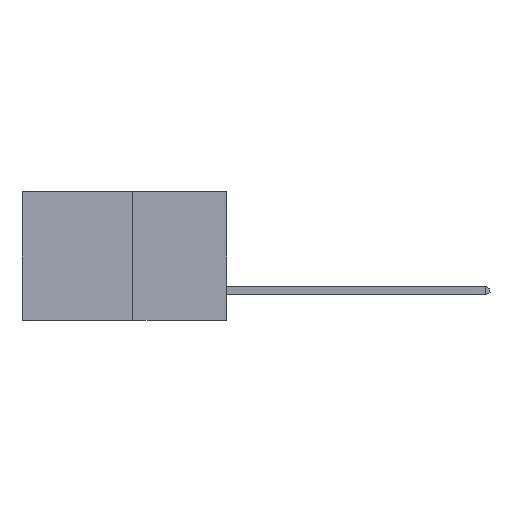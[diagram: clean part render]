
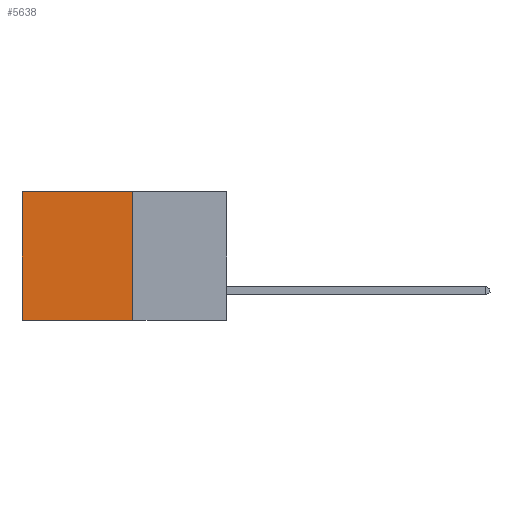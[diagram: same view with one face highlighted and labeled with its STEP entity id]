
A CAD part, left-side view. The second image highlights one B-rep face of the part: STEP entity #5638.
In plain terms, the highlighted planar face has unit normal (-1, 0, 0).
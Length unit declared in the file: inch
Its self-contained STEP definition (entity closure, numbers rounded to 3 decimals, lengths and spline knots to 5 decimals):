
#57 = FACE_OUTER_BOUND ( 'NONE', #10405, .T. ) ;
#211 = CARTESIAN_POINT ( 'NONE',  ( 0.277, 0.59, 0. ) ) ;
#411 = VERTEX_POINT ( 'NONE', #783 ) ;
#620 = CARTESIAN_POINT ( 'NONE',  ( 0.277, 0.27, -0.37 ) ) ;
#766 = AXIS2_PLACEMENT_3D ( 'NONE', #9885, #10184, #10251 ) ;
#783 = CARTESIAN_POINT ( 'NONE',  ( 0.277, 0.59, -0.37 ) ) ;
#1372 = EDGE_CURVE ( 'NONE', #1798, #411, #10619, .T. ) ;
#1446 = ORIENTED_EDGE ( 'NONE', *, *, #6670, .T. ) ;
#1680 = EDGE_CURVE ( 'NONE', #7975, #7936, #5465, .T. ) ;
#1716 = DIRECTION ( 'NONE',  ( 0., 1., 0. ) ) ;
#1798 = VERTEX_POINT ( 'NONE', #6508 ) ;
#1836 = ORIENTED_EDGE ( 'NONE', *, *, #1372, .F. ) ;
#1842 = ORIENTED_EDGE ( 'NONE', *, *, #2317, .F. ) ;
#2160 = VECTOR ( 'NONE', #1716, 39.37008 ) ;
#2317 = EDGE_CURVE ( 'NONE', #7975, #1798, #6098, .T. ) ;
#2874 = LINE ( 'NONE', #5718, #9077 ) ;
#3230 = VECTOR ( 'NONE', #9500, 39.37008 ) ;
#3699 = DIRECTION ( 'NONE',  ( 0., 0., -1. ) ) ;
#4056 = ORIENTED_EDGE ( 'NONE', *, *, #1680, .T. ) ;
#4765 = CARTESIAN_POINT ( 'NONE',  ( 0.277, 0.27, 0. ) ) ;
#5465 = LINE ( 'NONE', #9347, #3230 ) ;
#5638 = ADVANCED_FACE ( 'NONE', ( #57 ), #9644, .F. ) ;
#5678 = DIRECTION ( 'NONE',  ( 0., 0., -1. ) ) ;
#5718 = CARTESIAN_POINT ( 'NONE',  ( 0.277, 0.59, -0.37 ) ) ;
#5899 = CARTESIAN_POINT ( 'NONE',  ( 0.277, 0.27, -0.37 ) ) ;
#6098 = LINE ( 'NONE', #620, #8089 ) ;
#6508 = CARTESIAN_POINT ( 'NONE',  ( 0.277, 0.27, -0.37 ) ) ;
#6670 = EDGE_CURVE ( 'NONE', #7936, #411, #2874, .T. ) ;
#7936 = VERTEX_POINT ( 'NONE', #211 ) ;
#7975 = VERTEX_POINT ( 'NONE', #4765 ) ;
#8089 = VECTOR ( 'NONE', #3699, 39.37008 ) ;
#9077 = VECTOR ( 'NONE', #5678, 39.37008 ) ;
#9347 = CARTESIAN_POINT ( 'NONE',  ( 0.277, 0.27, 0. ) ) ;
#9500 = DIRECTION ( 'NONE',  ( 0., 1., 0. ) ) ;
#9644 = PLANE ( 'NONE',  #766 ) ;
#9885 = CARTESIAN_POINT ( 'NONE',  ( 0.277, 0.27, -0.37 ) ) ;
#10184 = DIRECTION ( 'NONE',  ( 1., 0., 0. ) ) ;
#10251 = DIRECTION ( 'NONE',  ( 0., 0., -1. ) ) ;
#10405 = EDGE_LOOP ( 'NONE', ( #1446, #1836, #1842, #4056 ) ) ;
#10619 = LINE ( 'NONE', #5899, #2160 ) ;
